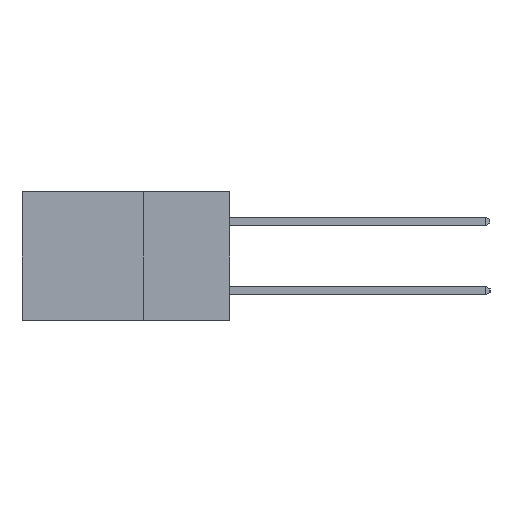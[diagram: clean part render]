
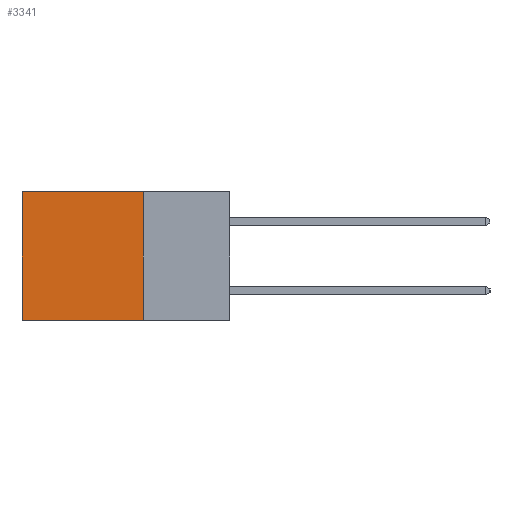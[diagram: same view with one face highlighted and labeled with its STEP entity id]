
A CAD part, left-side view. The second image highlights one B-rep face of the part: STEP entity #3341.
In plain terms, the highlighted planar face has unit normal (-1, 0, 0).
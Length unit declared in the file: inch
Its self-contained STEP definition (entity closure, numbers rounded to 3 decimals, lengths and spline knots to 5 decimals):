
#1396 = VECTOR ( 'NONE', #7095, 39.37008 ) ;
#1473 = CARTESIAN_POINT ( 'NONE',  ( 0.2615, 0.6, 0. ) ) ;
#1769 = VERTEX_POINT ( 'NONE', #6240 ) ;
#2001 = VECTOR ( 'NONE', #5516, 39.37008 ) ;
#2218 = LINE ( 'NONE', #5310, #7720 ) ;
#2221 = VERTEX_POINT ( 'NONE', #6239 ) ;
#2618 = ORIENTED_EDGE ( 'NONE', *, *, #7052, .T. ) ;
#3341 = ADVANCED_FACE ( 'NONE', ( #7004 ), #4389, .F. ) ;
#4003 = CARTESIAN_POINT ( 'NONE',  ( 0.2615, 0.25, 0. ) ) ;
#4219 = LINE ( 'NONE', #4003, #1396 ) ;
#4364 = DIRECTION ( 'NONE',  ( 0., 0., -1. ) ) ;
#4376 = DIRECTION ( 'NONE',  ( 1., 0., 0. ) ) ;
#4389 = PLANE ( 'NONE',  #8087 ) ;
#4468 = DIRECTION ( 'NONE',  ( 0., 0., -1. ) ) ;
#4485 = CARTESIAN_POINT ( 'NONE',  ( 0.2615, 0.25, -0.37 ) ) ;
#5073 = EDGE_CURVE ( 'NONE', #2221, #5390, #2218, .T. ) ;
#5310 = CARTESIAN_POINT ( 'NONE',  ( 0.2615, 0.25, -0.37 ) ) ;
#5362 = DIRECTION ( 'NONE',  ( 0., 1., 0. ) ) ;
#5390 = VERTEX_POINT ( 'NONE', #12471 ) ;
#5516 = DIRECTION ( 'NONE',  ( 0., 0., -1. ) ) ;
#5590 = VECTOR ( 'NONE', #4468, 39.37008 ) ;
#6239 = CARTESIAN_POINT ( 'NONE',  ( 0.2615, 0.25, -0.37 ) ) ;
#6240 = CARTESIAN_POINT ( 'NONE',  ( 0.2615, 0.25, 0. ) ) ;
#6637 = ORIENTED_EDGE ( 'NONE', *, *, #5073, .F. ) ;
#7004 = FACE_OUTER_BOUND ( 'NONE', #9024, .T. ) ;
#7052 = EDGE_CURVE ( 'NONE', #10636, #5390, #8169, .T. ) ;
#7095 = DIRECTION ( 'NONE',  ( 0., 1., 0. ) ) ;
#7241 = EDGE_CURVE ( 'NONE', #1769, #2221, #13316, .T. ) ;
#7523 = CARTESIAN_POINT ( 'NONE',  ( 0.2615, 0.6, -0.37 ) ) ;
#7720 = VECTOR ( 'NONE', #5362, 39.37008 ) ;
#7970 = ORIENTED_EDGE ( 'NONE', *, *, #12651, .T. ) ;
#8087 = AXIS2_PLACEMENT_3D ( 'NONE', #8904, #4376, #4364 ) ;
#8169 = LINE ( 'NONE', #7523, #2001 ) ;
#8904 = CARTESIAN_POINT ( 'NONE',  ( 0.2615, 0.25, -0.37 ) ) ;
#9024 = EDGE_LOOP ( 'NONE', ( #2618, #6637, #11619, #7970 ) ) ;
#10636 = VERTEX_POINT ( 'NONE', #1473 ) ;
#11619 = ORIENTED_EDGE ( 'NONE', *, *, #7241, .F. ) ;
#12471 = CARTESIAN_POINT ( 'NONE',  ( 0.2615, 0.6, -0.37 ) ) ;
#12651 = EDGE_CURVE ( 'NONE', #1769, #10636, #4219, .T. ) ;
#13316 = LINE ( 'NONE', #4485, #5590 ) ;
